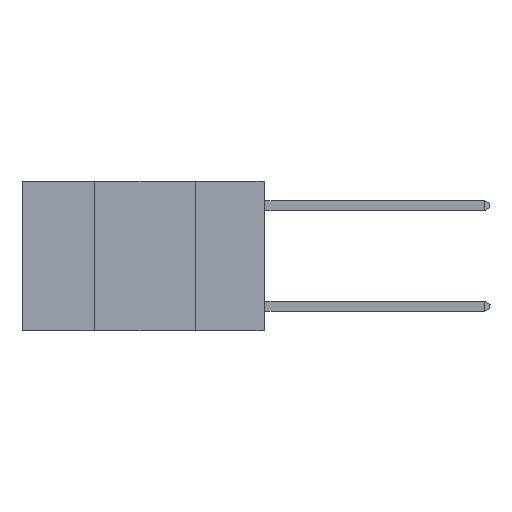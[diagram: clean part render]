
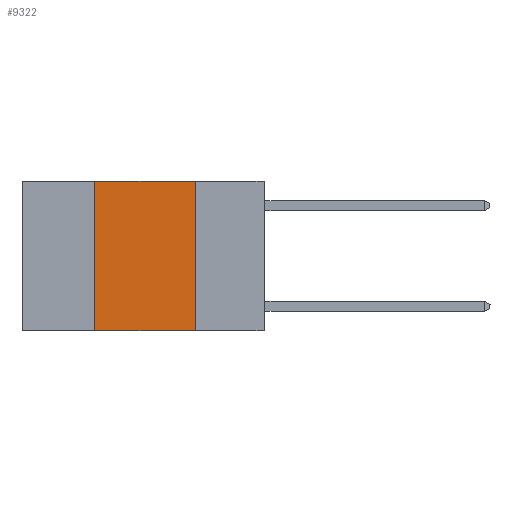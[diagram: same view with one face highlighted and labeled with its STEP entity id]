
A CAD part, left-side view. The second image highlights one B-rep face of the part: STEP entity #9322.
In plain terms, the highlighted planar face has unit normal (-1, 0, 0).
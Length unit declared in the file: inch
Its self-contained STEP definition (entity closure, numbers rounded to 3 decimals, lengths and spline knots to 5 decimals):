
#88 = CARTESIAN_POINT ( 'NONE',  ( 0., 0.42, -0.37 ) ) ;
#444 = EDGE_CURVE ( 'NONE', #2414, #15479, #8019, .T. ) ;
#681 = CARTESIAN_POINT ( 'NONE',  ( 0., 0.42, 0. ) ) ;
#1258 = FACE_OUTER_BOUND ( 'NONE', #16852, .T. ) ;
#2111 = CARTESIAN_POINT ( 'NONE',  ( 0., 0.17, -0.37 ) ) ;
#2287 = DIRECTION ( 'NONE',  ( 0., 0., -1. ) ) ;
#2414 = VERTEX_POINT ( 'NONE', #88 ) ;
#2984 = CARTESIAN_POINT ( 'NONE',  ( 0., 0.17, 0. ) ) ;
#3213 = EDGE_CURVE ( 'NONE', #2414, #19677, #6828, .T. ) ;
#3234 = CARTESIAN_POINT ( 'NONE',  ( 0., 0.42, 0. ) ) ;
#3898 = ORIENTED_EDGE ( 'NONE', *, *, #444, .T. ) ;
#4560 = LINE ( 'NONE', #16710, #7738 ) ;
#5069 = DIRECTION ( 'NONE',  ( 1., 0., 0. ) ) ;
#5169 = CARTESIAN_POINT ( 'NONE',  ( 0., 0.6, -0.37 ) ) ;
#6512 = AXIS2_PLACEMENT_3D ( 'NONE', #9711, #5069, #16033 ) ;
#6828 = LINE ( 'NONE', #681, #10486 ) ;
#7512 = VECTOR ( 'NONE', #12614, 39.37008 ) ;
#7738 = VECTOR ( 'NONE', #15160, 39.37008 ) ;
#8019 = LINE ( 'NONE', #5169, #7512 ) ;
#8961 = EDGE_CURVE ( 'NONE', #19677, #12153, #4560, .T. ) ;
#9322 = ADVANCED_FACE ( 'NONE', ( #1258 ), #14468, .F. ) ;
#9711 = CARTESIAN_POINT ( 'NONE',  ( 0., 0.6, 0. ) ) ;
#10486 = VECTOR ( 'NONE', #13334, 39.37008 ) ;
#10820 = EDGE_CURVE ( 'NONE', #12153, #15479, #11350, .T. ) ;
#11350 = LINE ( 'NONE', #11733, #11849 ) ;
#11733 = CARTESIAN_POINT ( 'NONE',  ( 0., 0.17, 0. ) ) ;
#11849 = VECTOR ( 'NONE', #2287, 39.37008 ) ;
#11964 = ORIENTED_EDGE ( 'NONE', *, *, #3213, .F. ) ;
#12153 = VERTEX_POINT ( 'NONE', #2984 ) ;
#12614 = DIRECTION ( 'NONE',  ( 0., -1., 0. ) ) ;
#13334 = DIRECTION ( 'NONE',  ( 0., 0., 1. ) ) ;
#14468 = PLANE ( 'NONE',  #6512 ) ;
#15160 = DIRECTION ( 'NONE',  ( 0., -1., 0. ) ) ;
#15479 = VERTEX_POINT ( 'NONE', #2111 ) ;
#16033 = DIRECTION ( 'NONE',  ( 0., 0., -1. ) ) ;
#16710 = CARTESIAN_POINT ( 'NONE',  ( 0., 0.6, 0. ) ) ;
#16852 = EDGE_LOOP ( 'NONE', ( #17274, #17836, #11964, #3898 ) ) ;
#17274 = ORIENTED_EDGE ( 'NONE', *, *, #10820, .F. ) ;
#17836 = ORIENTED_EDGE ( 'NONE', *, *, #8961, .F. ) ;
#19677 = VERTEX_POINT ( 'NONE', #3234 ) ;
